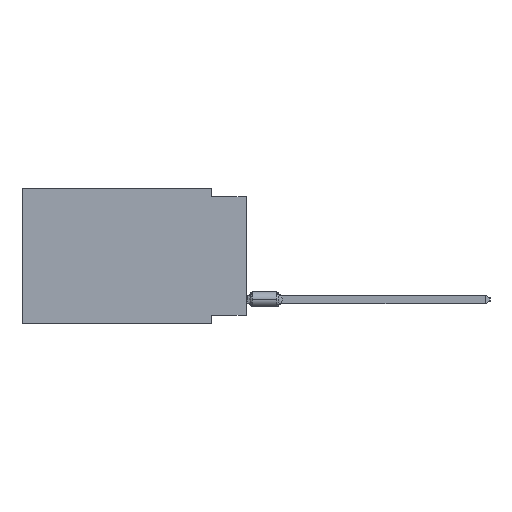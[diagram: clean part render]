
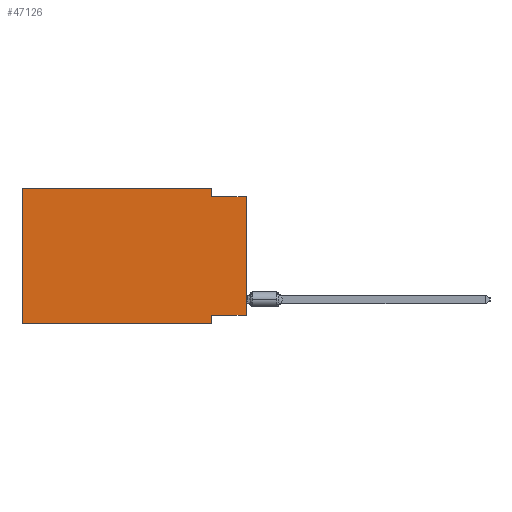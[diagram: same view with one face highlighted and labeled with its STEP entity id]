
A CAD part, left-side view. The second image highlights one B-rep face of the part: STEP entity #47126.
In plain terms, the highlighted planar face has unit normal (-1, 0, 0).
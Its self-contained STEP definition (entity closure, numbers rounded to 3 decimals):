
#839 = LINE ( 'NONE', #50618, #54278 ) ;
#1569 = VECTOR ( 'NONE', #64028, 1000. ) ;
#2201 = EDGE_CURVE ( 'NONE', #27967, #2653, #23664, .T. ) ;
#2653 = VERTEX_POINT ( 'NONE', #41266 ) ;
#3072 = EDGE_CURVE ( 'NONE', #41540, #9128, #57345, .T. ) ;
#3359 = CARTESIAN_POINT ( 'NONE',  ( 0., 16.383, -9.906 ) ) ;
#3587 = EDGE_CURVE ( 'NONE', #64179, #2653, #42194, .T. ) ;
#3649 = CARTESIAN_POINT ( 'NONE',  ( 0., 16.383, 0. ) ) ;
#5649 = ORIENTED_EDGE ( 'NONE', *, *, #21178, .F. ) ;
#7707 = VECTOR ( 'NONE', #67731, 1000. ) ;
#9128 = VERTEX_POINT ( 'NONE', #37353 ) ;
#9532 = ORIENTED_EDGE ( 'NONE', *, *, #16371, .F. ) ;
#10084 = VECTOR ( 'NONE', #66955, 1000. ) ;
#13924 = CARTESIAN_POINT ( 'NONE',  ( 0., 0., 0. ) ) ;
#14130 = CARTESIAN_POINT ( 'NONE',  ( 0., 16.383, -9.906 ) ) ;
#16156 = LINE ( 'NONE', #66654, #39490 ) ;
#16371 = EDGE_CURVE ( 'NONE', #65658, #49985, #29307, .T. ) ;
#17807 = EDGE_CURVE ( 'NONE', #53951, #49985, #19615, .T. ) ;
#18318 = DIRECTION ( 'NONE',  ( 0., 0., -1. ) ) ;
#19615 = LINE ( 'NONE', #13924, #1569 ) ;
#20709 = ORIENTED_EDGE ( 'NONE', *, *, #68476, .F. ) ;
#21178 = EDGE_CURVE ( 'NONE', #53951, #27967, #24348, .T. ) ;
#22897 = ORIENTED_EDGE ( 'NONE', *, *, #17807, .T. ) ;
#23180 = CARTESIAN_POINT ( 'NONE',  ( 0., 0., -0.635 ) ) ;
#23574 = DIRECTION ( 'NONE',  ( 0., 0., 1. ) ) ;
#23656 = DIRECTION ( 'NONE',  ( 1., 0., 0. ) ) ;
#23664 = LINE ( 'NONE', #57081, #31773 ) ;
#24348 = LINE ( 'NONE', #46034, #7707 ) ;
#27967 = VERTEX_POINT ( 'NONE', #51383 ) ;
#29307 = LINE ( 'NONE', #50669, #51521 ) ;
#31773 = VECTOR ( 'NONE', #67760, 1000. ) ;
#32530 = AXIS2_PLACEMENT_3D ( 'NONE', #67035, #23656, #18318 ) ;
#34999 = DIRECTION ( 'NONE',  ( 0., -1., 0. ) ) ;
#35140 = CARTESIAN_POINT ( 'NONE',  ( 0., 0., -9.271 ) ) ;
#37353 = CARTESIAN_POINT ( 'NONE',  ( 0., 2.54, 0. ) ) ;
#37666 = ORIENTED_EDGE ( 'NONE', *, *, #3587, .T. ) ;
#39490 = VECTOR ( 'NONE', #40692, 1000. ) ;
#40692 = DIRECTION ( 'NONE',  ( 0., 0., -1. ) ) ;
#41266 = CARTESIAN_POINT ( 'NONE',  ( 0., 2.54, -9.906 ) ) ;
#41540 = VERTEX_POINT ( 'NONE', #48973 ) ;
#42194 = LINE ( 'NONE', #14130, #47653 ) ;
#43325 = ORIENTED_EDGE ( 'NONE', *, *, #2201, .F. ) ;
#46034 = CARTESIAN_POINT ( 'NONE',  ( 0., 0., -9.271 ) ) ;
#47126 = ADVANCED_FACE ( 'NONE', ( #62403 ), #56366, .F. ) ;
#47653 = VECTOR ( 'NONE', #52871, 1000. ) ;
#48973 = CARTESIAN_POINT ( 'NONE',  ( 0., 16.383, 0. ) ) ;
#49985 = VERTEX_POINT ( 'NONE', #23180 ) ;
#50618 = CARTESIAN_POINT ( 'NONE',  ( 0., 16.383, 0. ) ) ;
#50669 = CARTESIAN_POINT ( 'NONE',  ( 0., 0., -0.635 ) ) ;
#50771 = EDGE_CURVE ( 'NONE', #9128, #65658, #16156, .T. ) ;
#51134 = ORIENTED_EDGE ( 'NONE', *, *, #3072, .F. ) ;
#51383 = CARTESIAN_POINT ( 'NONE',  ( 0., 2.54, -9.271 ) ) ;
#51521 = VECTOR ( 'NONE', #34999, 1000. ) ;
#52871 = DIRECTION ( 'NONE',  ( 0., -1., 0. ) ) ;
#53951 = VERTEX_POINT ( 'NONE', #35140 ) ;
#54278 = VECTOR ( 'NONE', #23574, 1000. ) ;
#56366 = PLANE ( 'NONE',  #32530 ) ;
#56607 = CARTESIAN_POINT ( 'NONE',  ( 0., 2.54, -0.635 ) ) ;
#57081 = CARTESIAN_POINT ( 'NONE',  ( 0., 2.54, -9.906 ) ) ;
#57345 = LINE ( 'NONE', #3649, #10084 ) ;
#62403 = FACE_OUTER_BOUND ( 'NONE', #68559, .T. ) ;
#64028 = DIRECTION ( 'NONE',  ( 0., 0., 1. ) ) ;
#64179 = VERTEX_POINT ( 'NONE', #3359 ) ;
#65328 = ORIENTED_EDGE ( 'NONE', *, *, #50771, .F. ) ;
#65658 = VERTEX_POINT ( 'NONE', #56607 ) ;
#66654 = CARTESIAN_POINT ( 'NONE',  ( 0., 2.54, 0. ) ) ;
#66955 = DIRECTION ( 'NONE',  ( 0., -1., 0. ) ) ;
#67035 = CARTESIAN_POINT ( 'NONE',  ( 0., 16.383, 0. ) ) ;
#67731 = DIRECTION ( 'NONE',  ( 0., 1., 0. ) ) ;
#67760 = DIRECTION ( 'NONE',  ( 0., 0., -1. ) ) ;
#68476 = EDGE_CURVE ( 'NONE', #64179, #41540, #839, .T. ) ;
#68559 = EDGE_LOOP ( 'NONE', ( #22897, #9532, #65328, #51134, #20709, #37666, #43325, #5649 ) ) ;
